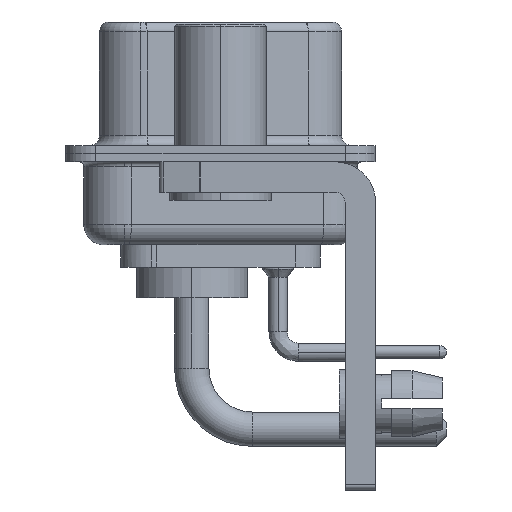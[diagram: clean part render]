
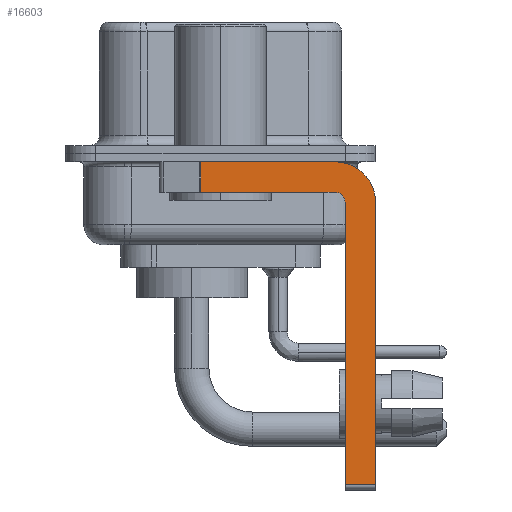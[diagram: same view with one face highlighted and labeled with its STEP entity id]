
A CAD part, left-side view. The second image highlights one B-rep face of the part: STEP entity #16603.
In plain terms, the highlighted planar face has unit normal (-1, 0, 0).
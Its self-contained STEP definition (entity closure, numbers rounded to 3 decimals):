
#257 = ORIENTED_EDGE ( 'NONE', *, *, #5979, .F. ) ;
#328 = DIRECTION ( 'NONE',  ( 0., 0., -1. ) ) ;
#412 = AXIS2_PLACEMENT_3D ( 'NONE', #4514, #21550, #328 ) ;
#462 = EDGE_CURVE ( 'NONE', #11651, #23776, #25929, .T. ) ;
#475 = PLANE ( 'NONE',  #412 ) ;
#584 = DIRECTION ( 'NONE',  ( 0., 0., 1. ) ) ;
#850 = EDGE_CURVE ( 'NONE', #17708, #8942, #17245, .T. ) ;
#877 = CARTESIAN_POINT ( 'NONE',  ( -2.9, -7.65, -16.35 ) ) ;
#988 = CARTESIAN_POINT ( 'NONE',  ( -2.9, -5.65, -1.9 ) ) ;
#1137 = ORIENTED_EDGE ( 'NONE', *, *, #26290, .F. ) ;
#1797 = VERTEX_POINT ( 'NONE', #877 ) ;
#2013 = CARTESIAN_POINT ( 'NONE',  ( -2.9, -5.65, -1.9 ) ) ;
#2089 = VERTEX_POINT ( 'NONE', #19021 ) ;
#2176 = VECTOR ( 'NONE', #27369, 1000. ) ;
#3536 = DIRECTION ( 'NONE',  ( 1., 0., 0. ) ) ;
#3871 = VERTEX_POINT ( 'NONE', #4602 ) ;
#4485 = EDGE_CURVE ( 'NONE', #3871, #7715, #20229, .T. ) ;
#4514 = CARTESIAN_POINT ( 'NONE',  ( -2.9, -5.65, -2.4 ) ) ;
#4602 = CARTESIAN_POINT ( 'NONE',  ( -2.9, -6.15, -2.4 ) ) ;
#5081 = EDGE_CURVE ( 'NONE', #2089, #1797, #9576, .T. ) ;
#5155 = LINE ( 'NONE', #9051, #9741 ) ;
#5280 = VECTOR ( 'NONE', #6931, 1000. ) ;
#5979 = EDGE_CURVE ( 'NONE', #7715, #23776, #19708, .T. ) ;
#6244 = ORIENTED_EDGE ( 'NONE', *, *, #17279, .F. ) ;
#6376 = CARTESIAN_POINT ( 'NONE',  ( -2.9, -5.65, -2.4 ) ) ;
#6931 = DIRECTION ( 'NONE',  ( 0., 0., -1. ) ) ;
#7351 = CARTESIAN_POINT ( 'NONE',  ( -2.9, 0.978, -0.4 ) ) ;
#7715 = VERTEX_POINT ( 'NONE', #2013 ) ;
#7952 = AXIS2_PLACEMENT_3D ( 'NONE', #9617, #3536, #16145 ) ;
#8051 = VECTOR ( 'NONE', #20688, 1000. ) ;
#8828 = VECTOR ( 'NONE', #22199, 1000. ) ;
#8942 = VERTEX_POINT ( 'NONE', #16039 ) ;
#9051 = CARTESIAN_POINT ( 'NONE',  ( -2.9, -6.15, -16.6 ) ) ;
#9468 = CARTESIAN_POINT ( 'NONE',  ( -2.9, 0.978, -1.9 ) ) ;
#9576 = LINE ( 'NONE', #9716, #12750 ) ;
#9617 = CARTESIAN_POINT ( 'NONE',  ( -2.9, -5.65, -2.4 ) ) ;
#9716 = CARTESIAN_POINT ( 'NONE',  ( -2.9, -5.65, -16.35 ) ) ;
#9741 = VECTOR ( 'NONE', #584, 1000. ) ;
#10302 = LINE ( 'NONE', #22647, #8051 ) ;
#10972 = ORIENTED_EDGE ( 'NONE', *, *, #850, .F. ) ;
#11153 = EDGE_LOOP ( 'NONE', ( #1137, #22287, #257, #13777, #6244, #14203, #20670, #10972 ) ) ;
#11223 = CARTESIAN_POINT ( 'NONE',  ( -2.9, 0.978, -1.9 ) ) ;
#11651 = VERTEX_POINT ( 'NONE', #7351 ) ;
#12750 = VECTOR ( 'NONE', #24688, 1000. ) ;
#13135 = DIRECTION ( 'NONE',  ( -1., 0., 0. ) ) ;
#13777 = ORIENTED_EDGE ( 'NONE', *, *, #4485, .F. ) ;
#14203 = ORIENTED_EDGE ( 'NONE', *, *, #5081, .T. ) ;
#16026 = CARTESIAN_POINT ( 'NONE',  ( -2.9, -5.65, -0.4 ) ) ;
#16039 = CARTESIAN_POINT ( 'NONE',  ( -2.9, -7.65, -2.4 ) ) ;
#16145 = DIRECTION ( 'NONE',  ( 0., 0., -1. ) ) ;
#16603 = ADVANCED_FACE ( 'NONE', ( #21424 ), #475, .F. ) ;
#16697 = LINE ( 'NONE', #19197, #2176 ) ;
#17245 = CIRCLE ( 'NONE', #7952, 2. ) ;
#17279 = EDGE_CURVE ( 'NONE', #2089, #3871, #5155, .T. ) ;
#17708 = VERTEX_POINT ( 'NONE', #16026 ) ;
#18472 = AXIS2_PLACEMENT_3D ( 'NONE', #6376, #13135, #19921 ) ;
#19021 = CARTESIAN_POINT ( 'NONE',  ( -2.9, -6.15, -16.35 ) ) ;
#19197 = CARTESIAN_POINT ( 'NONE',  ( -2.9, 3., -0.4 ) ) ;
#19708 = LINE ( 'NONE', #988, #8828 ) ;
#19921 = DIRECTION ( 'NONE',  ( 0., 0., 1. ) ) ;
#20229 = CIRCLE ( 'NONE', #18472, 0.5 ) ;
#20670 = ORIENTED_EDGE ( 'NONE', *, *, #21474, .F. ) ;
#20688 = DIRECTION ( 'NONE',  ( 0., 0., -1. ) ) ;
#21424 = FACE_OUTER_BOUND ( 'NONE', #11153, .T. ) ;
#21474 = EDGE_CURVE ( 'NONE', #8942, #1797, #10302, .T. ) ;
#21550 = DIRECTION ( 'NONE',  ( 1., 0., 0. ) ) ;
#22199 = DIRECTION ( 'NONE',  ( 0., 1., 0. ) ) ;
#22287 = ORIENTED_EDGE ( 'NONE', *, *, #462, .T. ) ;
#22647 = CARTESIAN_POINT ( 'NONE',  ( -2.9, -7.65, -2.4 ) ) ;
#23776 = VERTEX_POINT ( 'NONE', #9468 ) ;
#24688 = DIRECTION ( 'NONE',  ( 0., -1., 0. ) ) ;
#25929 = LINE ( 'NONE', #11223, #5280 ) ;
#26290 = EDGE_CURVE ( 'NONE', #11651, #17708, #16697, .T. ) ;
#27369 = DIRECTION ( 'NONE',  ( 0., -1., 0. ) ) ;
